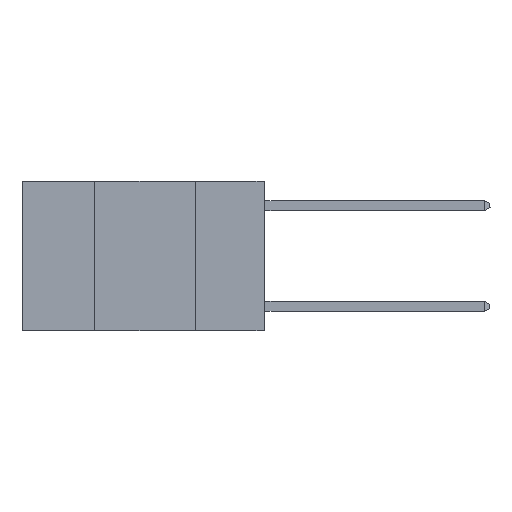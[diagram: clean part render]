
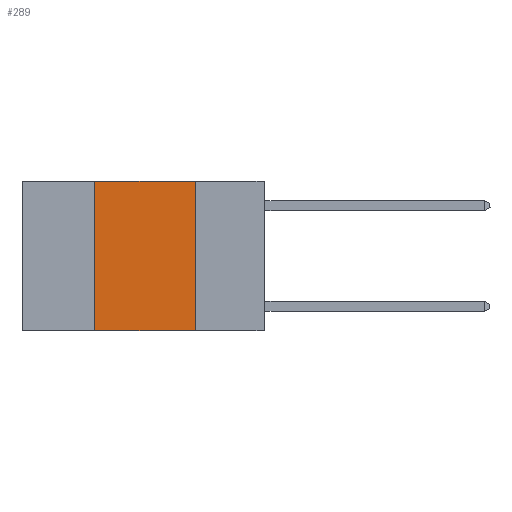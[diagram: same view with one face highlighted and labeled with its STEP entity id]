
A CAD part, left-side view. The second image highlights one B-rep face of the part: STEP entity #289.
In plain terms, the highlighted planar face has unit normal (-1, 0, 0).
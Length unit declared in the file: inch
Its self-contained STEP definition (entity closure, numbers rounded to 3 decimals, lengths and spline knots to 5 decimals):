
#289 = ADVANCED_FACE ( 'NONE', ( #6981 ), #4807, .F. ) ;
#327 = CARTESIAN_POINT ( 'NONE',  ( 0., 0.6, -0.37 ) ) ;
#974 = ORIENTED_EDGE ( 'NONE', *, *, #8246, .T. ) ;
#1332 = CARTESIAN_POINT ( 'NONE',  ( 0., 0.42, 0. ) ) ;
#1670 = CARTESIAN_POINT ( 'NONE',  ( 0., 0.6, 0. ) ) ;
#2026 = LINE ( 'NONE', #2995, #9030 ) ;
#2392 = VECTOR ( 'NONE', #6807, 39.37008 ) ;
#2438 = VERTEX_POINT ( 'NONE', #6788 ) ;
#2542 = EDGE_CURVE ( 'NONE', #4973, #5181, #8072, .T. ) ;
#2570 = DIRECTION ( 'NONE',  ( 0., 0., -1. ) ) ;
#2844 = ORIENTED_EDGE ( 'NONE', *, *, #2542, .F. ) ;
#2995 = CARTESIAN_POINT ( 'NONE',  ( 0., 0.42, 0. ) ) ;
#3894 = EDGE_LOOP ( 'NONE', ( #2844, #8810, #3974, #974 ) ) ;
#3974 = ORIENTED_EDGE ( 'NONE', *, *, #6339, .F. ) ;
#4061 = AXIS2_PLACEMENT_3D ( 'NONE', #6605, #7677, #2570 ) ;
#4807 = PLANE ( 'NONE',  #4061 ) ;
#4811 = VECTOR ( 'NONE', #6751, 39.37008 ) ;
#4973 = VERTEX_POINT ( 'NONE', #5566 ) ;
#5181 = VERTEX_POINT ( 'NONE', #9251 ) ;
#5566 = CARTESIAN_POINT ( 'NONE',  ( 0., 0.17, 0. ) ) ;
#6074 = VECTOR ( 'NONE', #8884, 39.37008 ) ;
#6339 = EDGE_CURVE ( 'NONE', #2438, #8427, #2026, .T. ) ;
#6453 = EDGE_CURVE ( 'NONE', #8427, #4973, #7107, .T. ) ;
#6605 = CARTESIAN_POINT ( 'NONE',  ( 0., 0.6, 0. ) ) ;
#6751 = DIRECTION ( 'NONE',  ( 0., -1., 0. ) ) ;
#6788 = CARTESIAN_POINT ( 'NONE',  ( 0., 0.42, -0.37 ) ) ;
#6807 = DIRECTION ( 'NONE',  ( 0., 0., -1. ) ) ;
#6965 = CARTESIAN_POINT ( 'NONE',  ( 0., 0.17, 0. ) ) ;
#6981 = FACE_OUTER_BOUND ( 'NONE', #3894, .T. ) ;
#7107 = LINE ( 'NONE', #1670, #4811 ) ;
#7677 = DIRECTION ( 'NONE',  ( 1., 0., 0. ) ) ;
#7825 = LINE ( 'NONE', #327, #6074 ) ;
#8072 = LINE ( 'NONE', #6965, #2392 ) ;
#8246 = EDGE_CURVE ( 'NONE', #2438, #5181, #7825, .T. ) ;
#8427 = VERTEX_POINT ( 'NONE', #1332 ) ;
#8586 = DIRECTION ( 'NONE',  ( 0., 0., 1. ) ) ;
#8810 = ORIENTED_EDGE ( 'NONE', *, *, #6453, .F. ) ;
#8884 = DIRECTION ( 'NONE',  ( 0., -1., 0. ) ) ;
#9030 = VECTOR ( 'NONE', #8586, 39.37008 ) ;
#9251 = CARTESIAN_POINT ( 'NONE',  ( 0., 0.17, -0.37 ) ) ;
